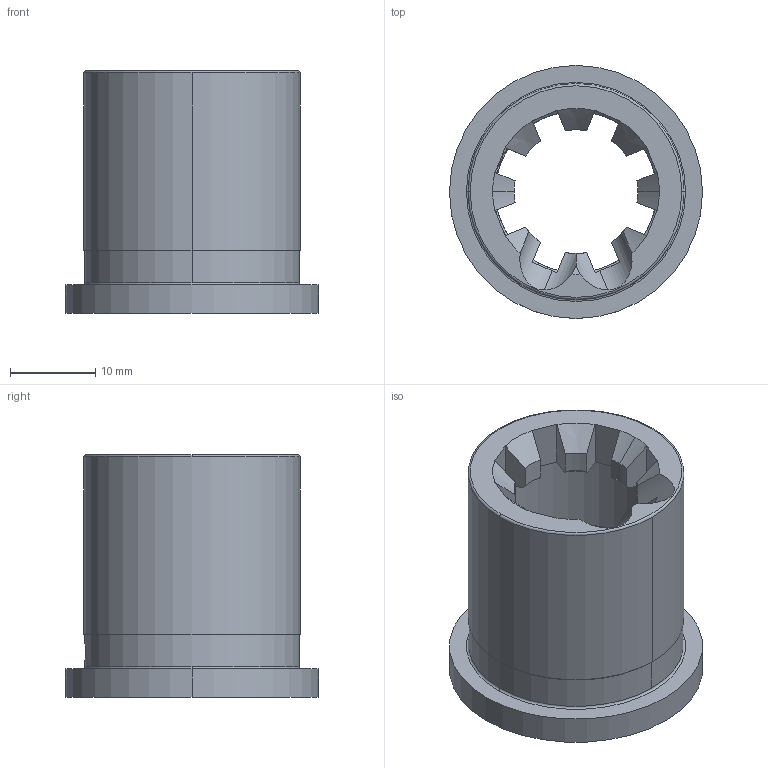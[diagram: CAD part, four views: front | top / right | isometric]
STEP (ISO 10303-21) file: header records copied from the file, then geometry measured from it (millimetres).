
FILE_DESCRIPTION (( 'STEP AP214' ), '1' );
FILE_NAME ('Barrel Extension.step.step', '2019-12-18T03:07:01', ( '' ), ( '' ), 'SwSTEP 2.0', 'SolidWorks 2019', '' );
FILE_SCHEMA (( 'AUTOMOTIVE_DESIGN' ));
Length unit declared in the file: millimetre
Products named in the file (1): Barrel Extension.step
Bounding box: 29.72 x 29.72 x 28.47 mm (x, y, z)
Volume: 6191.9 mm3; surface area: 5584.3 mm2
Topology: 1 solids, 1 shells, 117 faces, 318 edges, 204 vertices
Faces by surface type: cylinder 45, plane 30, cone 29, bspline 7, torus 6
Entity records: 5735 total; most frequent: CARTESIAN_POINT 3016, ORIENTED_EDGE 636, DIRECTION 492, EDGE_CURVE 318, VERTEX_POINT 204, AXIS2_PLACEMENT_3D 194, EDGE_LOOP 122, ADVANCED_FACE 117
